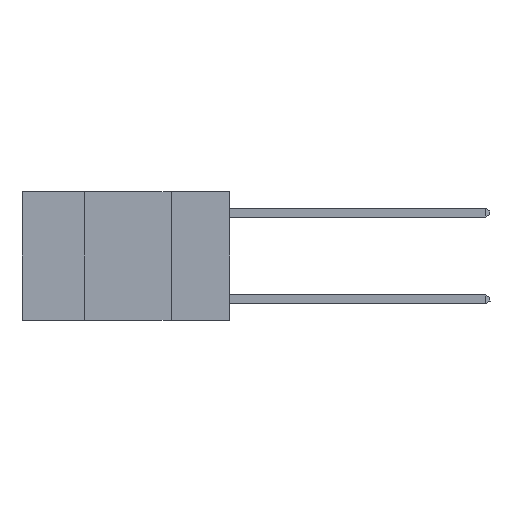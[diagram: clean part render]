
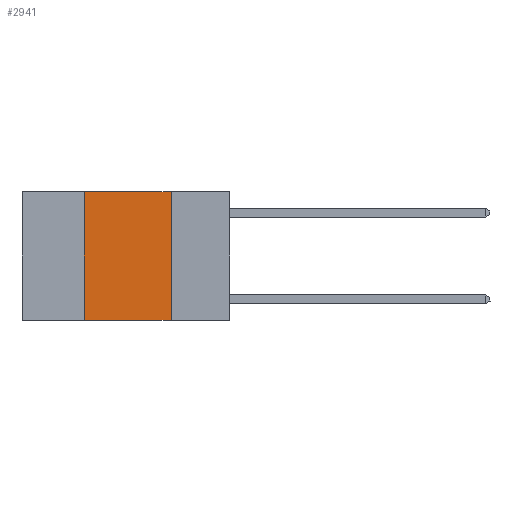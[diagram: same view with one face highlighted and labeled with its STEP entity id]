
A CAD part, left-side view. The second image highlights one B-rep face of the part: STEP entity #2941.
In plain terms, the highlighted planar face has unit normal (-1, 0, 0).
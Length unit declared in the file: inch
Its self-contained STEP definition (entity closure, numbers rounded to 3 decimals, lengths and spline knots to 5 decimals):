
#336 = DIRECTION ( 'NONE',  ( 1., 0., 0. ) ) ;
#539 = EDGE_CURVE ( 'NONE', #9214, #8779, #6619, .T. ) ;
#591 = CARTESIAN_POINT ( 'NONE',  ( 0., 0.17, 0. ) ) ;
#610 = VERTEX_POINT ( 'NONE', #3024 ) ;
#1497 = DIRECTION ( 'NONE',  ( 0., 0., -1. ) ) ;
#1628 = CARTESIAN_POINT ( 'NONE',  ( 0., 0.6, 0. ) ) ;
#2204 = CARTESIAN_POINT ( 'NONE',  ( 0., 0.6, -0.37 ) ) ;
#2385 = ORIENTED_EDGE ( 'NONE', *, *, #5877, .F. ) ;
#2389 = DIRECTION ( 'NONE',  ( 0., 0., 1. ) ) ;
#2465 = CARTESIAN_POINT ( 'NONE',  ( 0., 0.17, -0.37 ) ) ;
#2488 = ORIENTED_EDGE ( 'NONE', *, *, #8913, .F. ) ;
#2604 = VECTOR ( 'NONE', #1497, 39.37008 ) ;
#2733 = ORIENTED_EDGE ( 'NONE', *, *, #9322, .F. ) ;
#2941 = ADVANCED_FACE ( 'NONE', ( #5069 ), #9088, .F. ) ;
#3024 = CARTESIAN_POINT ( 'NONE',  ( 0., 0.42, 0. ) ) ;
#3384 = CARTESIAN_POINT ( 'NONE',  ( 0., 0.6, 0. ) ) ;
#3946 = VECTOR ( 'NONE', #7903, 39.37008 ) ;
#4183 = VECTOR ( 'NONE', #2389, 39.37008 ) ;
#4675 = AXIS2_PLACEMENT_3D ( 'NONE', #1628, #336, #9640 ) ;
#5069 = FACE_OUTER_BOUND ( 'NONE', #9334, .T. ) ;
#5877 = EDGE_CURVE ( 'NONE', #7998, #8779, #6635, .T. ) ;
#6619 = LINE ( 'NONE', #2204, #8550 ) ;
#6635 = LINE ( 'NONE', #8280, #2604 ) ;
#6796 = CARTESIAN_POINT ( 'NONE',  ( 0., 0.42, -0.37 ) ) ;
#7665 = CARTESIAN_POINT ( 'NONE',  ( 0., 0.42, 0. ) ) ;
#7903 = DIRECTION ( 'NONE',  ( 0., -1., 0. ) ) ;
#7922 = ORIENTED_EDGE ( 'NONE', *, *, #539, .T. ) ;
#7938 = LINE ( 'NONE', #3384, #3946 ) ;
#7998 = VERTEX_POINT ( 'NONE', #591 ) ;
#8280 = CARTESIAN_POINT ( 'NONE',  ( 0., 0.17, 0. ) ) ;
#8363 = LINE ( 'NONE', #7665, #4183 ) ;
#8550 = VECTOR ( 'NONE', #9132, 39.37008 ) ;
#8779 = VERTEX_POINT ( 'NONE', #2465 ) ;
#8913 = EDGE_CURVE ( 'NONE', #610, #7998, #7938, .T. ) ;
#9088 = PLANE ( 'NONE',  #4675 ) ;
#9132 = DIRECTION ( 'NONE',  ( 0., -1., 0. ) ) ;
#9214 = VERTEX_POINT ( 'NONE', #6796 ) ;
#9322 = EDGE_CURVE ( 'NONE', #9214, #610, #8363, .T. ) ;
#9334 = EDGE_LOOP ( 'NONE', ( #2385, #2488, #2733, #7922 ) ) ;
#9640 = DIRECTION ( 'NONE',  ( 0., 0., -1. ) ) ;
